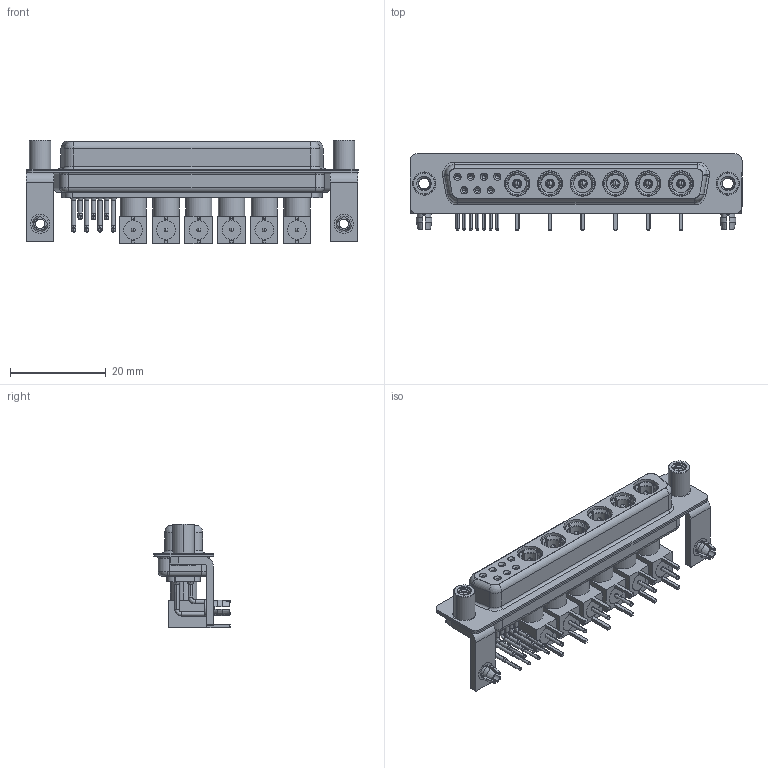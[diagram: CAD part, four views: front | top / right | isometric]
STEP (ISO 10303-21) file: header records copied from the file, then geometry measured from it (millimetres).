
FILE_DESCRIPTION (( 'STEP AP203' ), '1' );
FILE_NAME ('630-13W6240-7T5.STEP', '2022-06-03T12:53:50', ( '' ), ( '' ), 'SwSTEP 2.0', 'SolidWorks 2020', '' );
FILE_SCHEMA (( 'CONFIG_CONTROL_DESIGN' ));
Length unit declared in the file: millimetre
Products named in the file (21): 630Combo Shell Rear_37 Contacts; 630Combo Contact Row 1; 630Combo Housing_13W6; Insulator RA Pin; Co-Ax Plug Assy_RA; 630Combo Stabilizer Bracket; 630Combo Threaded Standoff_5; Co-Ax Plug_RA PC Tail; 630Combo Shell Front_37 Contacts; 630-13W6240-7T5; 630Combo Board Lock; RA Back Shell; Insulator Pin_Straight PC Tail; 630Combo Contact Row 2; Pin_RA; Locking Collar
Assembly tree (58 placements, depth 3):
  630-13W6240-7T5
    630Combo Housing_13W6
    630Combo Shell Front_37 Contacts
    630Combo Shell Rear_37 Contacts
    630Combo Stabilizer Bracket  x2
    630Combo Board Lock  x2
    630Combo Threaded Standoff_5  x2
    Co-Ax Plug Assy_RA
      Co-Ax Plug_RA PC Tail
      Insulator Pin_Straight PC Tail
      Pin_RA
      Locking Collar
      RA Back Shell
      Insulator RA Pin
    Co-Ax Plug Assy_RA
      Co-Ax Plug_RA PC Tail
      Insulator Pin_Straight PC Tail
      Pin_RA
      Locking Collar
      RA Back Shell
      Insulator RA Pin
    Co-Ax Plug Assy_RA
      Co-Ax Plug_RA PC Tail
      Insulator Pin_Straight PC Tail
      Pin_RA
      Locking Collar
      RA Back Shell
      Insulator RA Pin
    Co-Ax Plug Assy_RA
      Co-Ax Plug_RA PC Tail
      Insulator Pin_Straight PC Tail
      Pin_RA
      Locking Collar
      RA Back Shell
      Insulator RA Pin
    Co-Ax Plug Assy_RA
      Co-Ax Plug_RA PC Tail
      Insulator Pin_Straight PC Tail
      Pin_RA
      Locking Collar
      RA Back Shell
      Insulator RA Pin
    Co-Ax Plug Assy_RA
      Co-Ax Plug_RA PC Tail
      Insulator Pin_Straight PC Tail
      Pin_RA
      Locking Collar
      RA Back Shell
      Insulator RA Pin
    630Combo Contact Row 1  x4
    630Combo Contact Row 2  x3
Bounding box: 69.4 x 16 x 21.61 mm (x, y, z)
Volume: 7102.5 mm3; surface area: 17080.3 mm2
Topology: 52 solids, 52 shells, 1838 faces, 4520 edges, 2846 vertices
Faces by surface type: cylinder 780, plane 644, cone 257, torus 93, bspline 40, sphere 24
Entity records: 26345 total; most frequent: CARTESIAN_POINT 6064, DIRECTION 3859, ORIENTED_EDGE 3394, EDGE_CURVE 1697, AXIS2_PLACEMENT_3D 1566, VERTEX_POINT 1083, EDGE_LOOP 812, CIRCLE 811
